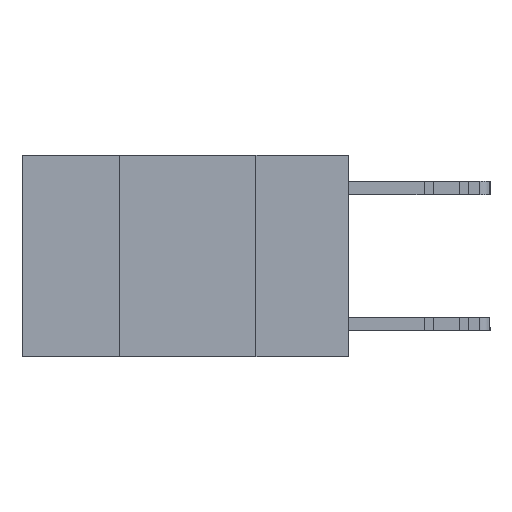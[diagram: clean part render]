
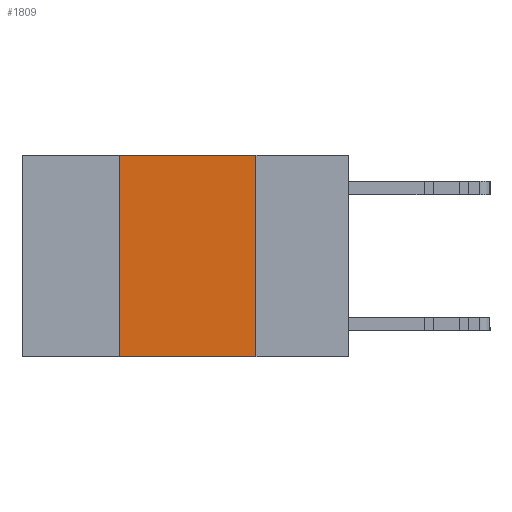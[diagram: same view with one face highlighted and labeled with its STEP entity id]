
A CAD part, left-side view. The second image highlights one B-rep face of the part: STEP entity #1809.
In plain terms, the highlighted planar face has unit normal (-1, 0, 0).
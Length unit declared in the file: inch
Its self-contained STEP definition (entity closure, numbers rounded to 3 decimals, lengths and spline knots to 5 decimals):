
#275 = DIRECTION ( 'NONE',  ( 0., -1., 0. ) ) ;
#1005 = CARTESIAN_POINT ( 'NONE',  ( 0., 0.17, 0. ) ) ;
#1809 = ADVANCED_FACE ( 'NONE', ( #22017 ), #17494, .F. ) ;
#2488 = VECTOR ( 'NONE', #14269, 39.37008 ) ;
#2771 = CARTESIAN_POINT ( 'NONE',  ( 0., 0.17, 0. ) ) ;
#3221 = VERTEX_POINT ( 'NONE', #25759 ) ;
#4453 = EDGE_CURVE ( 'NONE', #14978, #24425, #21627, .T. ) ;
#5315 = CARTESIAN_POINT ( 'NONE',  ( 0., 0.42, 0. ) ) ;
#5973 = EDGE_CURVE ( 'NONE', #3221, #24425, #20117, .T. ) ;
#7725 = LINE ( 'NONE', #5315, #23463 ) ;
#10055 = CARTESIAN_POINT ( 'NONE',  ( 0., 0.42, 0. ) ) ;
#10748 = DIRECTION ( 'NONE',  ( 1., 0., 0. ) ) ;
#11581 = VERTEX_POINT ( 'NONE', #10055 ) ;
#13735 = VECTOR ( 'NONE', #26741, 39.37008 ) ;
#13950 = EDGE_CURVE ( 'NONE', #11581, #14978, #18919, .T. ) ;
#14046 = ORIENTED_EDGE ( 'NONE', *, *, #13950, .F. ) ;
#14269 = DIRECTION ( 'NONE',  ( 0., 0., -1. ) ) ;
#14978 = VERTEX_POINT ( 'NONE', #2771 ) ;
#15892 = CARTESIAN_POINT ( 'NONE',  ( 0., 0.6, -0.37 ) ) ;
#17494 = PLANE ( 'NONE',  #28245 ) ;
#18163 = ORIENTED_EDGE ( 'NONE', *, *, #5973, .T. ) ;
#18919 = LINE ( 'NONE', #21182, #20449 ) ;
#18969 = DIRECTION ( 'NONE',  ( 0., 0., 1. ) ) ;
#19693 = EDGE_CURVE ( 'NONE', #3221, #11581, #7725, .T. ) ;
#19751 = CARTESIAN_POINT ( 'NONE',  ( 0., 0.6, 0. ) ) ;
#19821 = ORIENTED_EDGE ( 'NONE', *, *, #19693, .F. ) ;
#20117 = LINE ( 'NONE', #15892, #13735 ) ;
#20449 = VECTOR ( 'NONE', #275, 39.37008 ) ;
#21182 = CARTESIAN_POINT ( 'NONE',  ( 0., 0.6, 0. ) ) ;
#21627 = LINE ( 'NONE', #1005, #2488 ) ;
#22017 = FACE_OUTER_BOUND ( 'NONE', #27681, .T. ) ;
#23455 = CARTESIAN_POINT ( 'NONE',  ( 0., 0.17, -0.37 ) ) ;
#23463 = VECTOR ( 'NONE', #18969, 39.37008 ) ;
#24425 = VERTEX_POINT ( 'NONE', #23455 ) ;
#24726 = DIRECTION ( 'NONE',  ( 0., 0., -1. ) ) ;
#25469 = ORIENTED_EDGE ( 'NONE', *, *, #4453, .F. ) ;
#25759 = CARTESIAN_POINT ( 'NONE',  ( 0., 0.42, -0.37 ) ) ;
#26741 = DIRECTION ( 'NONE',  ( 0., -1., 0. ) ) ;
#27681 = EDGE_LOOP ( 'NONE', ( #25469, #14046, #19821, #18163 ) ) ;
#28245 = AXIS2_PLACEMENT_3D ( 'NONE', #19751, #10748, #24726 ) ;
